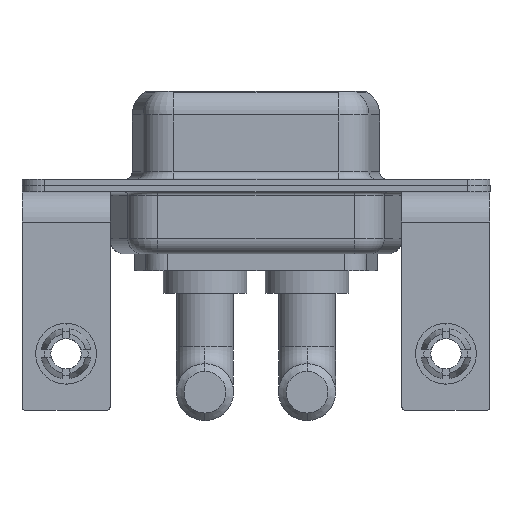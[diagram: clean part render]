
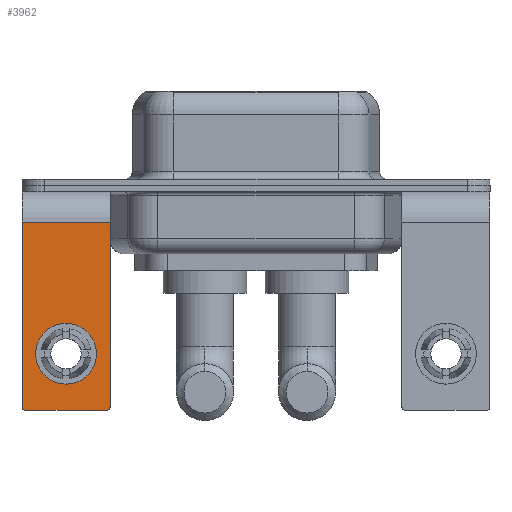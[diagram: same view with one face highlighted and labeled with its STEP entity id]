
A CAD part, front view. The second image highlights one B-rep face of the part: STEP entity #3962.
In plain terms, the highlighted planar face has unit normal (0, -1, 0).
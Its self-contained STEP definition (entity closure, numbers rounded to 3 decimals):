
#229 = CARTESIAN_POINT ( 'NONE',  ( 0., -6.25, -11.07 ) ) ;
#344 = CARTESIAN_POINT ( 'NONE',  ( -2.65, -6.25, -14.8 ) ) ;
#468 = VERTEX_POINT ( 'NONE', #9040 ) ;
#479 = DIRECTION ( 'NONE',  ( 0., 1., 0. ) ) ;
#556 = VERTEX_POINT ( 'NONE', #344 ) ;
#873 = EDGE_CURVE ( 'NONE', #468, #2902, #6891, .T. ) ;
#986 = ORIENTED_EDGE ( 'NONE', *, *, #3352, .T. ) ;
#1238 = DIRECTION ( 'NONE',  ( 0., 0., 1. ) ) ;
#1503 = ORIENTED_EDGE ( 'NONE', *, *, #873, .T. ) ;
#1583 = DIRECTION ( 'NONE',  ( 0., 0., 1. ) ) ;
#1834 = VECTOR ( 'NONE', #13707, 1000. ) ;
#1853 = ORIENTED_EDGE ( 'NONE', *, *, #12450, .T. ) ;
#1867 = EDGE_CURVE ( 'NONE', #2902, #556, #11027, .T. ) ;
#2096 = VECTOR ( 'NONE', #6240, 1000. ) ;
#2355 = ORIENTED_EDGE ( 'NONE', *, *, #13298, .F. ) ;
#2370 = LINE ( 'NONE', #13755, #7919 ) ;
#2815 = LINE ( 'NONE', #7304, #6103 ) ;
#2902 = VERTEX_POINT ( 'NONE', #12389 ) ;
#2951 = EDGE_CURVE ( 'NONE', #12078, #3371, #12306, .T. ) ;
#3057 = AXIS2_PLACEMENT_3D ( 'NONE', #14081, #479, #8434 ) ;
#3112 = ORIENTED_EDGE ( 'NONE', *, *, #2951, .T. ) ;
#3352 = EDGE_CURVE ( 'NONE', #3371, #12078, #12070, .T. ) ;
#3371 = VERTEX_POINT ( 'NONE', #13336 ) ;
#3638 = DIRECTION ( 'NONE',  ( 0., 1., 0. ) ) ;
#3862 = EDGE_LOOP ( 'NONE', ( #3112, #986 ) ) ;
#3958 = PLANE ( 'NONE',  #3057 ) ;
#3962 = ADVANCED_FACE ( 'NONE', ( #10487, #4907 ), #3958, .F. ) ;
#4456 = AXIS2_PLACEMENT_3D ( 'NONE', #11319, #12710, #1238 ) ;
#4518 = EDGE_LOOP ( 'NONE', ( #1503, #12521, #2355, #12629, #9889, #1853 ) ) ;
#4743 = CARTESIAN_POINT ( 'NONE',  ( 0., -6.25, -11.07 ) ) ;
#4907 = FACE_OUTER_BOUND ( 'NONE', #4518, .T. ) ;
#5014 = AXIS2_PLACEMENT_3D ( 'NONE', #4743, #3638, #8124 ) ;
#5095 = DIRECTION ( 'NONE',  ( -1., 0., 0. ) ) ;
#5755 = DIRECTION ( 'NONE',  ( 0., 0., 1. ) ) ;
#5978 = DIRECTION ( 'NONE',  ( 0., 0., -1. ) ) ;
#6025 = AXIS2_PLACEMENT_3D ( 'NONE', #11644, #9457, #1583 ) ;
#6103 = VECTOR ( 'NONE', #5095, 1000. ) ;
#6176 = VERTEX_POINT ( 'NONE', #9888 ) ;
#6240 = DIRECTION ( 'NONE',  ( -1., 0., 0. ) ) ;
#6891 = LINE ( 'NONE', #13426, #1834 ) ;
#7304 = CARTESIAN_POINT ( 'NONE',  ( 2.9, -6.25, -14.8 ) ) ;
#7919 = VECTOR ( 'NONE', #5978, 1000. ) ;
#8124 = DIRECTION ( 'NONE',  ( 0., 0., 1. ) ) ;
#8434 = DIRECTION ( 'NONE',  ( 0., 0., 1. ) ) ;
#9040 = CARTESIAN_POINT ( 'NONE',  ( -2.9, -6.25, -2.4 ) ) ;
#9457 = DIRECTION ( 'NONE',  ( 0., -1., 0. ) ) ;
#9477 = VERTEX_POINT ( 'NONE', #12948 ) ;
#9888 = CARTESIAN_POINT ( 'NONE',  ( 2.65, -6.25, -14.8 ) ) ;
#9889 = ORIENTED_EDGE ( 'NONE', *, *, #10668, .F. ) ;
#10163 = DIRECTION ( 'NONE',  ( 0., 1., 0. ) ) ;
#10487 = FACE_BOUND ( 'NONE', #3862, .T. ) ;
#10668 = EDGE_CURVE ( 'NONE', #10766, #9477, #2370, .T. ) ;
#10766 = VERTEX_POINT ( 'NONE', #13900 ) ;
#10944 = CARTESIAN_POINT ( 'NONE',  ( 2.9, -6.25, -2.4 ) ) ;
#11019 = LINE ( 'NONE', #10944, #2096 ) ;
#11027 = CIRCLE ( 'NONE', #4456, 0.25 ) ;
#11105 = CARTESIAN_POINT ( 'NONE',  ( 0., -6.25, -13.07 ) ) ;
#11319 = CARTESIAN_POINT ( 'NONE',  ( -2.65, -6.25, -14.55 ) ) ;
#11644 = CARTESIAN_POINT ( 'NONE',  ( 2.65, -6.25, -14.55 ) ) ;
#12070 = CIRCLE ( 'NONE', #13002, 2. ) ;
#12078 = VERTEX_POINT ( 'NONE', #11105 ) ;
#12306 = CIRCLE ( 'NONE', #5014, 2. ) ;
#12389 = CARTESIAN_POINT ( 'NONE',  ( -2.9, -6.25, -14.55 ) ) ;
#12450 = EDGE_CURVE ( 'NONE', #10766, #468, #11019, .T. ) ;
#12521 = ORIENTED_EDGE ( 'NONE', *, *, #1867, .T. ) ;
#12629 = ORIENTED_EDGE ( 'NONE', *, *, #13977, .T. ) ;
#12710 = DIRECTION ( 'NONE',  ( 0., -1., 0. ) ) ;
#12948 = CARTESIAN_POINT ( 'NONE',  ( 2.9, -6.25, -14.55 ) ) ;
#13002 = AXIS2_PLACEMENT_3D ( 'NONE', #229, #10163, #5755 ) ;
#13064 = CIRCLE ( 'NONE', #6025, 0.25 ) ;
#13298 = EDGE_CURVE ( 'NONE', #6176, #556, #2815, .T. ) ;
#13336 = CARTESIAN_POINT ( 'NONE',  ( 0., -6.25, -9.07 ) ) ;
#13426 = CARTESIAN_POINT ( 'NONE',  ( -2.9, -6.25, -2.4 ) ) ;
#13707 = DIRECTION ( 'NONE',  ( 0., 0., -1. ) ) ;
#13755 = CARTESIAN_POINT ( 'NONE',  ( 2.9, -6.25, -2.4 ) ) ;
#13900 = CARTESIAN_POINT ( 'NONE',  ( 2.9, -6.25, -2.4 ) ) ;
#13977 = EDGE_CURVE ( 'NONE', #6176, #9477, #13064, .T. ) ;
#14081 = CARTESIAN_POINT ( 'NONE',  ( 2.9, -6.25, -2.4 ) ) ;
